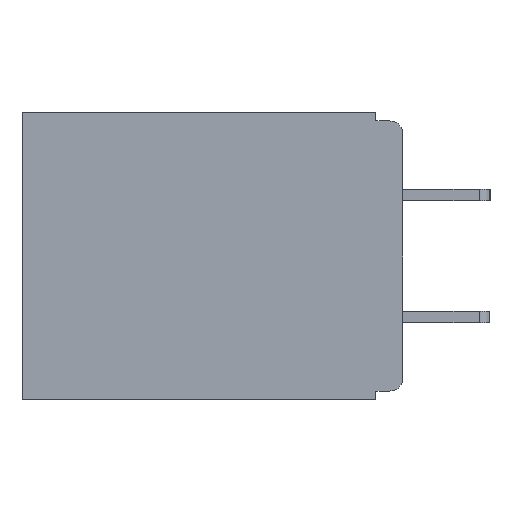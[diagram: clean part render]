
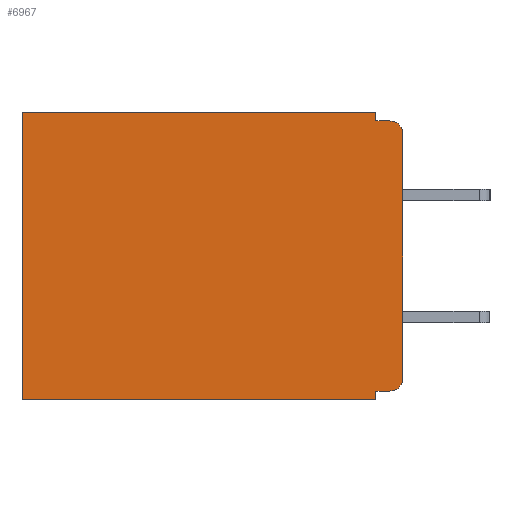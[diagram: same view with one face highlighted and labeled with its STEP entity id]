
A CAD part, left-side view. The second image highlights one B-rep face of the part: STEP entity #6967.
In plain terms, the highlighted planar face has unit normal (-1, 0, 0).
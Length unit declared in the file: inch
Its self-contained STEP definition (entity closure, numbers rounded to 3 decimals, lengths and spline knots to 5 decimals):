
#168 = VECTOR ( 'NONE', #679, 39.37008 ) ;
#581 = CARTESIAN_POINT ( 'NONE',  ( 0.3, 0.031, -0.01 ) ) ;
#679 = DIRECTION ( 'NONE',  ( 0., 0., -1. ) ) ;
#764 = FACE_OUTER_BOUND ( 'NONE', #13782, .T. ) ;
#938 = CARTESIAN_POINT ( 'NONE',  ( 0.3, 0., -0.33 ) ) ;
#970 = DIRECTION ( 'NONE',  ( 0., 0., -1. ) ) ;
#1016 = DIRECTION ( 'NONE',  ( 0., 0., -1. ) ) ;
#1055 = DIRECTION ( 'NONE',  ( 0., 0., -1. ) ) ;
#1323 = EDGE_CURVE ( 'NONE', #1618, #1700, #12720, .T. ) ;
#1493 = VERTEX_POINT ( 'NONE', #5096 ) ;
#1561 = VERTEX_POINT ( 'NONE', #581 ) ;
#1618 = VERTEX_POINT ( 'NONE', #12401 ) ;
#1700 = VERTEX_POINT ( 'NONE', #5650 ) ;
#1730 = EDGE_CURVE ( 'NONE', #1561, #10550, #12707, .T. ) ;
#1747 = VECTOR ( 'NONE', #6300, 39.37008 ) ;
#2032 = DIRECTION ( 'NONE',  ( 1., 0., 0. ) ) ;
#2124 = LINE ( 'NONE', #5110, #1747 ) ;
#2291 = LINE ( 'NONE', #13780, #14259 ) ;
#2444 = EDGE_CURVE ( 'NONE', #14597, #12608, #10345, .T. ) ;
#2692 = LINE ( 'NONE', #2942, #8909 ) ;
#2894 = ORIENTED_EDGE ( 'NONE', *, *, #13420, .F. ) ;
#2942 = CARTESIAN_POINT ( 'NONE',  ( 0.3, 0., -0.32 ) ) ;
#2981 = DIRECTION ( 'NONE',  ( 0., 1., 0. ) ) ;
#3348 = CARTESIAN_POINT ( 'NONE',  ( 0.3, 0.437, -0.33 ) ) ;
#3423 = VECTOR ( 'NONE', #5563, 39.37008 ) ;
#3559 = VERTEX_POINT ( 'NONE', #14243 ) ;
#4064 = EDGE_CURVE ( 'NONE', #1700, #1493, #9751, .T. ) ;
#4198 = ORIENTED_EDGE ( 'NONE', *, *, #4064, .T. ) ;
#4431 = ORIENTED_EDGE ( 'NONE', *, *, #2444, .F. ) ;
#4468 = ORIENTED_EDGE ( 'NONE', *, *, #1730, .F. ) ;
#5096 = CARTESIAN_POINT ( 'NONE',  ( 0.3, 0.437, -0.33 ) ) ;
#5110 = CARTESIAN_POINT ( 'NONE',  ( 0.3, 0., -0.33 ) ) ;
#5364 = ORIENTED_EDGE ( 'NONE', *, *, #14390, .T. ) ;
#5563 = DIRECTION ( 'NONE',  ( 0., -1., 0. ) ) ;
#5650 = CARTESIAN_POINT ( 'NONE',  ( 0.3, 0.437, 0. ) ) ;
#5905 = ORIENTED_EDGE ( 'NONE', *, *, #1323, .T. ) ;
#6068 = CARTESIAN_POINT ( 'NONE',  ( 0.3, 0.031, -0.32 ) ) ;
#6069 = CARTESIAN_POINT ( 'NONE',  ( 0.3, 0.015, -0.305 ) ) ;
#6165 = CIRCLE ( 'NONE', #6745, 0.015 ) ;
#6300 = DIRECTION ( 'NONE',  ( 0., 1., 0. ) ) ;
#6395 = LINE ( 'NONE', #7724, #168 ) ;
#6508 = ORIENTED_EDGE ( 'NONE', *, *, #8051, .F. ) ;
#6570 = VECTOR ( 'NONE', #2981, 39.37008 ) ;
#6701 = VECTOR ( 'NONE', #7469, 39.37008 ) ;
#6745 = AXIS2_PLACEMENT_3D ( 'NONE', #6069, #14143, #7254 ) ;
#6967 = ADVANCED_FACE ( 'NONE', ( #764 ), #11177, .F. ) ;
#7032 = CARTESIAN_POINT ( 'NONE',  ( 0.3, 0.015, -0.01 ) ) ;
#7254 = DIRECTION ( 'NONE',  ( 0., 0., -1. ) ) ;
#7462 = AXIS2_PLACEMENT_3D ( 'NONE', #938, #2032, #13686 ) ;
#7469 = DIRECTION ( 'NONE',  ( 0., 0., -1. ) ) ;
#7484 = AXIS2_PLACEMENT_3D ( 'NONE', #14882, #8040, #1016 ) ;
#7724 = CARTESIAN_POINT ( 'NONE',  ( 0.3, 0.031, 0. ) ) ;
#7873 = ORIENTED_EDGE ( 'NONE', *, *, #9169, .F. ) ;
#8040 = DIRECTION ( 'NONE',  ( -1., 0., 0. ) ) ;
#8051 = EDGE_CURVE ( 'NONE', #1618, #1561, #6395, .T. ) ;
#8909 = VECTOR ( 'NONE', #13397, 39.37008 ) ;
#9112 = CARTESIAN_POINT ( 'NONE',  ( 0.3, 0., -0.025 ) ) ;
#9169 = EDGE_CURVE ( 'NONE', #3559, #14597, #2692, .T. ) ;
#9580 = EDGE_CURVE ( 'NONE', #3559, #11574, #6165, .T. ) ;
#9751 = LINE ( 'NONE', #3348, #6701 ) ;
#10305 = CIRCLE ( 'NONE', #7484, 0.015 ) ;
#10345 = LINE ( 'NONE', #12315, #13049 ) ;
#10480 = EDGE_CURVE ( 'NONE', #13106, #11574, #2291, .T. ) ;
#10550 = VERTEX_POINT ( 'NONE', #7032 ) ;
#11177 = PLANE ( 'NONE',  #7462 ) ;
#11464 = CARTESIAN_POINT ( 'NONE',  ( 0.3, 0., 0. ) ) ;
#11574 = VERTEX_POINT ( 'NONE', #14596 ) ;
#12118 = CARTESIAN_POINT ( 'NONE',  ( 0.3, 0.031, -0.33 ) ) ;
#12315 = CARTESIAN_POINT ( 'NONE',  ( 0.3, 0.031, -0.33 ) ) ;
#12401 = CARTESIAN_POINT ( 'NONE',  ( 0.3, 0.031, 0. ) ) ;
#12442 = CARTESIAN_POINT ( 'NONE',  ( 0.3, 0., -0.01 ) ) ;
#12608 = VERTEX_POINT ( 'NONE', #12118 ) ;
#12707 = LINE ( 'NONE', #12442, #3423 ) ;
#12720 = LINE ( 'NONE', #11464, #6570 ) ;
#12991 = ORIENTED_EDGE ( 'NONE', *, *, #9580, .T. ) ;
#13049 = VECTOR ( 'NONE', #970, 39.37008 ) ;
#13106 = VERTEX_POINT ( 'NONE', #9112 ) ;
#13397 = DIRECTION ( 'NONE',  ( 0., 1., 0. ) ) ;
#13420 = EDGE_CURVE ( 'NONE', #12608, #1493, #2124, .T. ) ;
#13686 = DIRECTION ( 'NONE',  ( 0., 0., -1. ) ) ;
#13780 = CARTESIAN_POINT ( 'NONE',  ( 0.3, 0., -0.33 ) ) ;
#13782 = EDGE_LOOP ( 'NONE', ( #14879, #5364, #4468, #6508, #5905, #4198, #2894, #4431, #7873, #12991 ) ) ;
#14143 = DIRECTION ( 'NONE',  ( -1., 0., 0. ) ) ;
#14243 = CARTESIAN_POINT ( 'NONE',  ( 0.3, 0.015, -0.32 ) ) ;
#14259 = VECTOR ( 'NONE', #1055, 39.37008 ) ;
#14390 = EDGE_CURVE ( 'NONE', #13106, #10550, #10305, .T. ) ;
#14596 = CARTESIAN_POINT ( 'NONE',  ( 0.3, 0., -0.305 ) ) ;
#14597 = VERTEX_POINT ( 'NONE', #6068 ) ;
#14879 = ORIENTED_EDGE ( 'NONE', *, *, #10480, .F. ) ;
#14882 = CARTESIAN_POINT ( 'NONE',  ( 0.3, 0.015, -0.025 ) ) ;
